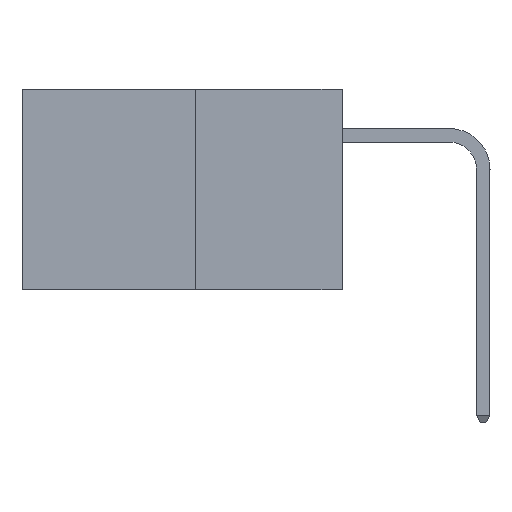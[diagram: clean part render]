
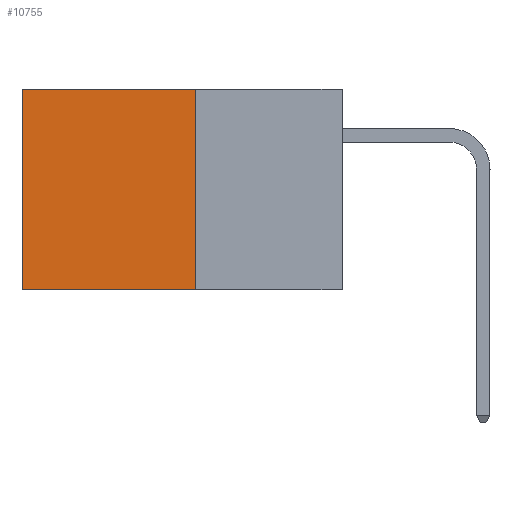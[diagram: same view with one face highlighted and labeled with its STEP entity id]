
A CAD part, left-side view. The second image highlights one B-rep face of the part: STEP entity #10755.
In plain terms, the highlighted planar face has unit normal (-1, 0, 0).
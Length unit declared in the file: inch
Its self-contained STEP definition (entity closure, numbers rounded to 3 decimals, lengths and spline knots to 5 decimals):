
#526 = VECTOR ( 'NONE', #1279, 39.37008 ) ;
#919 = VECTOR ( 'NONE', #7422, 39.37008 ) ;
#933 = LINE ( 'NONE', #3579, #14302 ) ;
#1279 = DIRECTION ( 'NONE',  ( 0., 1., 0. ) ) ;
#1770 = CARTESIAN_POINT ( 'NONE',  ( 0.277, 0.27, 0. ) ) ;
#3579 = CARTESIAN_POINT ( 'NONE',  ( 0.277, 0.59, -0.37 ) ) ;
#3868 = CARTESIAN_POINT ( 'NONE',  ( 0.277, 0.27, -0.37 ) ) ;
#4011 = LINE ( 'NONE', #12994, #526 ) ;
#4399 = LINE ( 'NONE', #9980, #919 ) ;
#5161 = ORIENTED_EDGE ( 'NONE', *, *, #16445, .T. ) ;
#5442 = PLANE ( 'NONE',  #13071 ) ;
#5946 = ORIENTED_EDGE ( 'NONE', *, *, #12464, .F. ) ;
#6460 = DIRECTION ( 'NONE',  ( 0., 0., -1. ) ) ;
#6779 = EDGE_CURVE ( 'NONE', #7564, #15657, #4011, .T. ) ;
#7135 = CARTESIAN_POINT ( 'NONE',  ( 0.277, 0.59, -0.37 ) ) ;
#7237 = EDGE_CURVE ( 'NONE', #12083, #8920, #4399, .T. ) ;
#7422 = DIRECTION ( 'NONE',  ( 0., 1., 0. ) ) ;
#7564 = VERTEX_POINT ( 'NONE', #15832 ) ;
#7973 = ORIENTED_EDGE ( 'NONE', *, *, #7237, .T. ) ;
#8068 = DIRECTION ( 'NONE',  ( 0., 0., -1. ) ) ;
#8920 = VERTEX_POINT ( 'NONE', #9416 ) ;
#9416 = CARTESIAN_POINT ( 'NONE',  ( 0.277, 0.59, 0. ) ) ;
#9931 = VECTOR ( 'NONE', #6460, 39.37008 ) ;
#9980 = CARTESIAN_POINT ( 'NONE',  ( 0.277, 0.27, 0. ) ) ;
#10755 = ADVANCED_FACE ( 'NONE', ( #15184 ), #5442, .F. ) ;
#10850 = ORIENTED_EDGE ( 'NONE', *, *, #6779, .F. ) ;
#11031 = EDGE_LOOP ( 'NONE', ( #5161, #10850, #5946, #7973 ) ) ;
#11396 = DIRECTION ( 'NONE',  ( 0., 0., -1. ) ) ;
#12083 = VERTEX_POINT ( 'NONE', #1770 ) ;
#12464 = EDGE_CURVE ( 'NONE', #12083, #7564, #12968, .T. ) ;
#12968 = LINE ( 'NONE', #3868, #9931 ) ;
#12994 = CARTESIAN_POINT ( 'NONE',  ( 0.277, 0.27, -0.37 ) ) ;
#13071 = AXIS2_PLACEMENT_3D ( 'NONE', #14468, #15757, #8068 ) ;
#14302 = VECTOR ( 'NONE', #11396, 39.37008 ) ;
#14468 = CARTESIAN_POINT ( 'NONE',  ( 0.277, 0.27, -0.37 ) ) ;
#15184 = FACE_OUTER_BOUND ( 'NONE', #11031, .T. ) ;
#15657 = VERTEX_POINT ( 'NONE', #7135 ) ;
#15757 = DIRECTION ( 'NONE',  ( 1., 0., 0. ) ) ;
#15832 = CARTESIAN_POINT ( 'NONE',  ( 0.277, 0.27, -0.37 ) ) ;
#16445 = EDGE_CURVE ( 'NONE', #8920, #15657, #933, .T. ) ;
